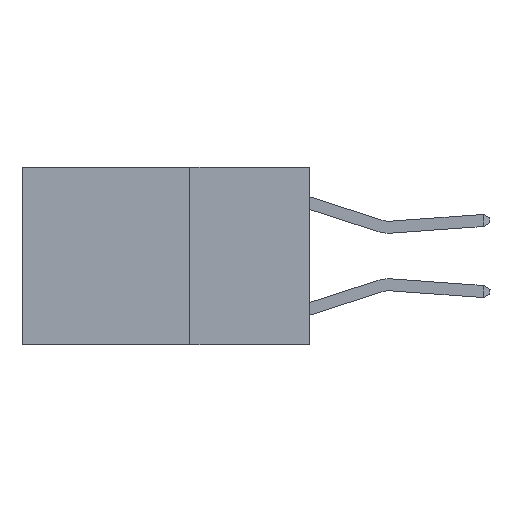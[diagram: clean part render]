
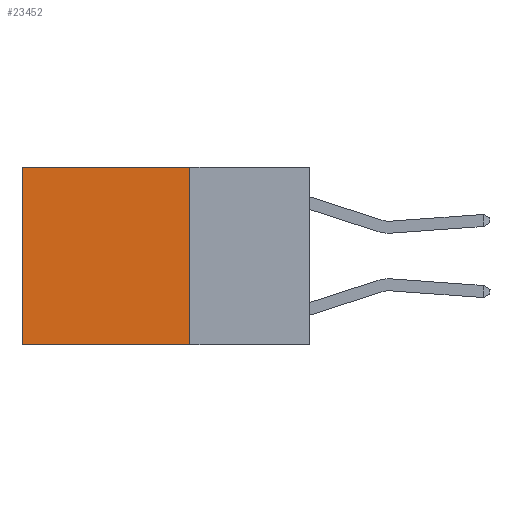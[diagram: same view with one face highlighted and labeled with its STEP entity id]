
A CAD part, left-side view. The second image highlights one B-rep face of the part: STEP entity #23452.
In plain terms, the highlighted planar face has unit normal (-1, 0, 0).
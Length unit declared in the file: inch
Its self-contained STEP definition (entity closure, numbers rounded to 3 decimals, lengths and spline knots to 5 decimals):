
#105 = CARTESIAN_POINT ( 'NONE',  ( 0.2625, 0.25, 0. ) ) ;
#492 = EDGE_CURVE ( 'NONE', #19192, #17182, #7852, .T. ) ;
#940 = ORIENTED_EDGE ( 'NONE', *, *, #8095, .T. ) ;
#1195 = AXIS2_PLACEMENT_3D ( 'NONE', #23071, #25251, #12199 ) ;
#3450 = PLANE ( 'NONE',  #1195 ) ;
#4268 = DIRECTION ( 'NONE',  ( 0., 1., 0. ) ) ;
#4708 = ORIENTED_EDGE ( 'NONE', *, *, #5394, .T. ) ;
#4904 = VECTOR ( 'NONE', #5521, 39.37008 ) ;
#5394 = EDGE_CURVE ( 'NONE', #10822, #17182, #10674, .T. ) ;
#5521 = DIRECTION ( 'NONE',  ( 0., 0., -1. ) ) ;
#5765 = CARTESIAN_POINT ( 'NONE',  ( 0.2625, 0.25, -0.37 ) ) ;
#6230 = EDGE_LOOP ( 'NONE', ( #4708, #18714, #17385, #940 ) ) ;
#7581 = EDGE_CURVE ( 'NONE', #22475, #19192, #7882, .T. ) ;
#7852 = LINE ( 'NONE', #5765, #13648 ) ;
#7882 = LINE ( 'NONE', #105, #11590 ) ;
#8095 = EDGE_CURVE ( 'NONE', #22475, #10822, #16731, .T. ) ;
#8342 = CARTESIAN_POINT ( 'NONE',  ( 0.2625, 0.25, 0. ) ) ;
#10121 = CARTESIAN_POINT ( 'NONE',  ( 0.2625, 0.6, -0.37 ) ) ;
#10674 = LINE ( 'NONE', #18549, #4904 ) ;
#10822 = VERTEX_POINT ( 'NONE', #21796 ) ;
#11382 = CARTESIAN_POINT ( 'NONE',  ( 0.2625, 0.25, 0. ) ) ;
#11590 = VECTOR ( 'NONE', #17619, 39.37008 ) ;
#12199 = DIRECTION ( 'NONE',  ( 0., 0., -1. ) ) ;
#13648 = VECTOR ( 'NONE', #4268, 39.37008 ) ;
#14884 = DIRECTION ( 'NONE',  ( 0., 1., 0. ) ) ;
#16031 = VECTOR ( 'NONE', #14884, 39.37008 ) ;
#16731 = LINE ( 'NONE', #8342, #16031 ) ;
#17182 = VERTEX_POINT ( 'NONE', #10121 ) ;
#17385 = ORIENTED_EDGE ( 'NONE', *, *, #7581, .F. ) ;
#17619 = DIRECTION ( 'NONE',  ( 0., 0., -1. ) ) ;
#18549 = CARTESIAN_POINT ( 'NONE',  ( 0.2625, 0.6, 0. ) ) ;
#18714 = ORIENTED_EDGE ( 'NONE', *, *, #492, .F. ) ;
#19192 = VERTEX_POINT ( 'NONE', #23059 ) ;
#21796 = CARTESIAN_POINT ( 'NONE',  ( 0.2625, 0.6, 0. ) ) ;
#22212 = FACE_OUTER_BOUND ( 'NONE', #6230, .T. ) ;
#22475 = VERTEX_POINT ( 'NONE', #11382 ) ;
#23059 = CARTESIAN_POINT ( 'NONE',  ( 0.2625, 0.25, -0.37 ) ) ;
#23071 = CARTESIAN_POINT ( 'NONE',  ( 0.2625, 0.25, 0. ) ) ;
#23452 = ADVANCED_FACE ( 'NONE', ( #22212 ), #3450, .F. ) ;
#25251 = DIRECTION ( 'NONE',  ( 1., 0., 0. ) ) ;
